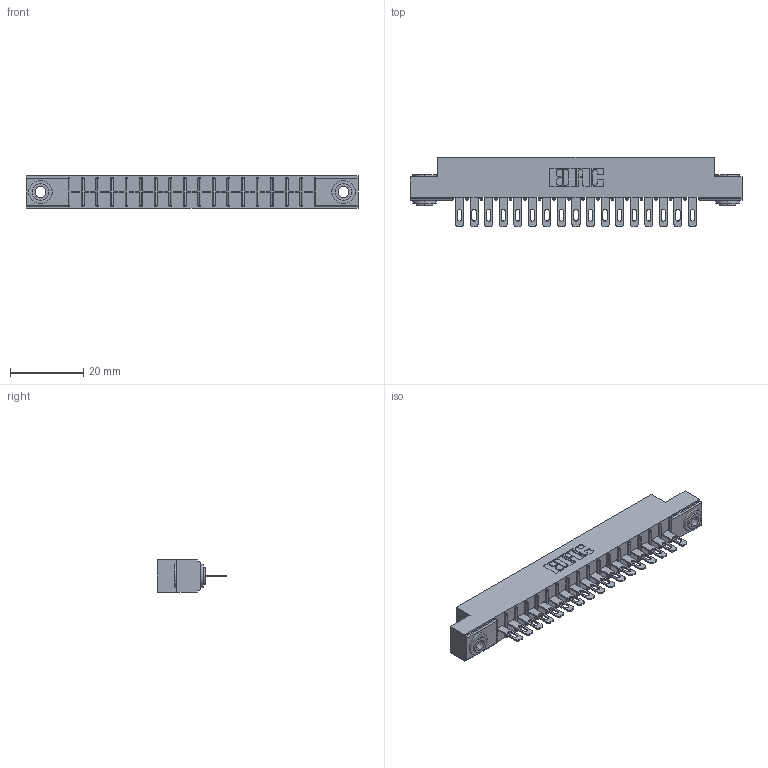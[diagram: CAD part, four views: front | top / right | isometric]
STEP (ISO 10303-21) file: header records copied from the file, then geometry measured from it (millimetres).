
FILE_DESCRIPTION (( 'STEP AP203' ), '1' );
FILE_NAME ('316-017-400-103.STEP', '2020-09-22T18:02:31', ( '' ), ( '' ), 'SwSTEP 2.0', 'SolidWorks 2020', '' );
FILE_SCHEMA (( 'CONFIG_CONTROL_DESIGN' ));
Length unit declared in the file: inch
Products named in the file (4): 306 Part_.156 Dia; 345-250-002_345-250-002-102; 306-290-001_100; 316-017-400-103
Assembly tree (20 placements, depth 2):
  316-017-400-103
    306 Part_.156 Dia
    306-290-001_100  x17
    345-250-002_345-250-002-102  x2
Bounding box: 90.37 x 18.87 x 8.71 mm (x, y, z)
Volume: 6218.7 mm3; surface area: 9550.7 mm2
Topology: 20 solids, 20 shells, 1460 faces, 4083 edges, 2626 vertices
Faces by surface type: plane 942, cylinder 442, sphere 68, cone 8
Entity records: 20321 total; most frequent: CARTESIAN_POINT 3387, DIRECTION 3357, ORIENTED_EDGE 3346, EDGE_CURVE 1673, LINE 1285, VECTOR 1285, VERTEX_POINT 1066, AXIS2_PLACEMENT_3D 1036
